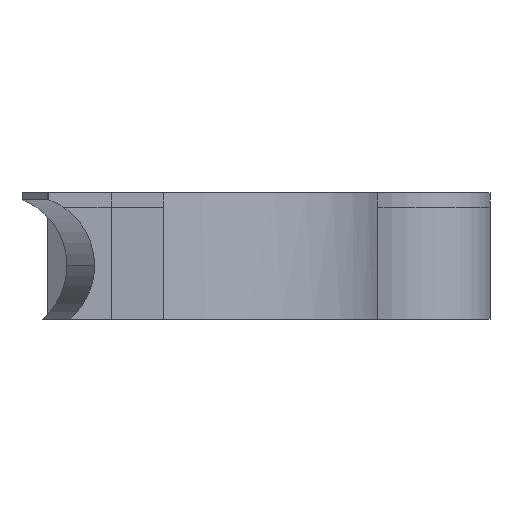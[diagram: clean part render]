
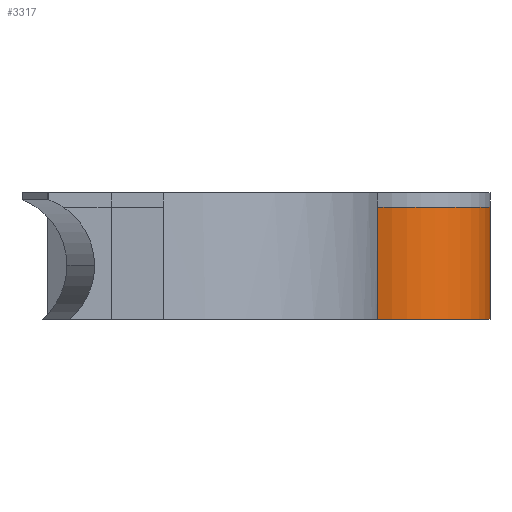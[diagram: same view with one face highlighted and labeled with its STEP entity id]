
A CAD part, left-side view. The second image highlights one B-rep face of the part: STEP entity #3317.
In plain terms, the highlighted cylindrical face has radius 6 mm (diameter 12 mm), a partial arc.
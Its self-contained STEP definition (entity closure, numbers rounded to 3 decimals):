
#795 = VERTEX_POINT('',#796);
#796 = CARTESIAN_POINT('',(42.343,0.,0.)
  );
#847 = PLANE('',#848);
#848 = AXIS2_PLACEMENT_3D('',#849,#850,#851);
#849 = CARTESIAN_POINT('',(0.,0.,0.));
#850 = DIRECTION('',(0.,1.,0.));
#851 = DIRECTION('',(1.,0.,0.));
#1685 = VERTEX_POINT('',#1686);
#1686 = CARTESIAN_POINT('',(42.343,0.,8.));
#1707 = EDGE_CURVE('',#795,#1685,#1708,.T.);
#1708 = SURFACE_CURVE('',#1709,(#1713,#1719),.PCURVE_S1.);
#1709 = LINE('',#1710,#1711);
#1710 = CARTESIAN_POINT('',(42.343,0.,8.));
#1711 = VECTOR('',#1712,1.);
#1712 = DIRECTION('',(0.,0.,1.));
#1713 = PCURVE('',#847,#1714);
#1714 = DEFINITIONAL_REPRESENTATION('',(#1715),#1718);
#1715 = B_SPLINE_CURVE_WITH_KNOTS('',1,(#1716,#1717),.UNSPECIFIED.,.F.,
  .F.,(2,2),(-8.,0.),.PIECEWISE_BEZIER_KNOTS.);
#1716 = CARTESIAN_POINT('',(42.343,0.));
#1717 = CARTESIAN_POINT('',(42.343,-8.));
#1718 = ( GEOMETRIC_REPRESENTATION_CONTEXT(2) 
PARAMETRIC_REPRESENTATION_CONTEXT() REPRESENTATION_CONTEXT('2D SPACE',''
  ) );
#1719 = PCURVE('',#1720,#1725);
#1720 = CYLINDRICAL_SURFACE('',#1721,6.);
#1721 = AXIS2_PLACEMENT_3D('',#1722,#1723,#1724);
#1722 = CARTESIAN_POINT('',(48.,-2.,8.));
#1723 = DIRECTION('',(0.,0.,1.));
#1724 = DIRECTION('',(1.,0.,0.));
#1725 = DEFINITIONAL_REPRESENTATION('',(#1726),#1729);
#1726 = B_SPLINE_CURVE_WITH_KNOTS('',1,(#1727,#1728),.UNSPECIFIED.,.F.,
  .F.,(2,2),(-8.,0.),.PIECEWISE_BEZIER_KNOTS.);
#1727 = CARTESIAN_POINT('',(2.802,-8.));
#1728 = CARTESIAN_POINT('',(2.802,0.));
#1729 = ( GEOMETRIC_REPRESENTATION_CONTEXT(2) 
PARAMETRIC_REPRESENTATION_CONTEXT() REPRESENTATION_CONTEXT('2D SPACE',''
  ) );
#1843 = PLANE('',#1844);
#1844 = AXIS2_PLACEMENT_3D('',#1845,#1846,#1847);
#1845 = CARTESIAN_POINT('',(54.,-2.,0.));
#1846 = DIRECTION('',(0.,0.,-1.));
#1847 = DIRECTION('',(-1.,0.,0.));
#2028 = CYLINDRICAL_SURFACE('',#2029,6.);
#2029 = AXIS2_PLACEMENT_3D('',#2030,#2031,#2032);
#2030 = CARTESIAN_POINT('',(48.,-2.,8.));
#2031 = DIRECTION('',(0.,0.,1.));
#2032 = DIRECTION('',(1.,0.,0.));
#2433 = CYLINDRICAL_SURFACE('',#2434,6.);
#2434 = AXIS2_PLACEMENT_3D('',#2435,#2436,#2437);
#2435 = CARTESIAN_POINT('',(48.,-2.,8.));
#2436 = DIRECTION('',(0.,0.,-1.));
#2437 = DIRECTION('',(1.,0.,0.));
#3317 = ADVANCED_FACE('',(#3318),#1720,.T.);
#3318 = FACE_BOUND('',#3319,.T.);
#3319 = EDGE_LOOP('',(#3320,#3345,#3367,#3368));
#3320 = ORIENTED_EDGE('',*,*,#3321,.F.);
#3321 = EDGE_CURVE('',#3322,#3324,#3326,.T.);
#3322 = VERTEX_POINT('',#3323);
#3323 = CARTESIAN_POINT('',(54.,-2.,8.));
#3324 = VERTEX_POINT('',#3325);
#3325 = CARTESIAN_POINT('',(54.,-2.,0.));
#3326 = SURFACE_CURVE('',#3327,(#3331,#3338),.PCURVE_S1.);
#3327 = LINE('',#3328,#3329);
#3328 = CARTESIAN_POINT('',(54.,-2.,8.));
#3329 = VECTOR('',#3330,1.);
#3330 = DIRECTION('',(0.,0.,-1.));
#3331 = PCURVE('',#1720,#3332);
#3332 = DEFINITIONAL_REPRESENTATION('',(#3333),#3337);
#3333 = LINE('',#3334,#3335);
#3334 = CARTESIAN_POINT('',(6.283,0.));
#3335 = VECTOR('',#3336,1.);
#3336 = DIRECTION('',(0.,-1.));
#3337 = ( GEOMETRIC_REPRESENTATION_CONTEXT(2) 
PARAMETRIC_REPRESENTATION_CONTEXT() REPRESENTATION_CONTEXT('2D SPACE',''
  ) );
#3338 = PCURVE('',#2028,#3339);
#3339 = DEFINITIONAL_REPRESENTATION('',(#3340),#3344);
#3340 = LINE('',#3341,#3342);
#3341 = CARTESIAN_POINT('',(0.,0.));
#3342 = VECTOR('',#3343,1.);
#3343 = DIRECTION('',(0.,-1.));
#3344 = ( GEOMETRIC_REPRESENTATION_CONTEXT(2) 
PARAMETRIC_REPRESENTATION_CONTEXT() REPRESENTATION_CONTEXT('2D SPACE',''
  ) );
#3345 = ORIENTED_EDGE('',*,*,#3346,.F.);
#3346 = EDGE_CURVE('',#1685,#3322,#3347,.T.);
#3347 = SURFACE_CURVE('',#3348,(#3353,#3360),.PCURVE_S1.);
#3348 = CIRCLE('',#3349,6.);
#3349 = AXIS2_PLACEMENT_3D('',#3350,#3351,#3352);
#3350 = CARTESIAN_POINT('',(48.,-2.,8.));
#3351 = DIRECTION('',(0.,0.,1.));
#3352 = DIRECTION('',(1.,0.,0.));
#3353 = PCURVE('',#1720,#3354);
#3354 = DEFINITIONAL_REPRESENTATION('',(#3355),#3359);
#3355 = LINE('',#3356,#3357);
#3356 = CARTESIAN_POINT('',(0.,0.));
#3357 = VECTOR('',#3358,1.);
#3358 = DIRECTION('',(1.,0.));
#3359 = ( GEOMETRIC_REPRESENTATION_CONTEXT(2) 
PARAMETRIC_REPRESENTATION_CONTEXT() REPRESENTATION_CONTEXT('2D SPACE',''
  ) );
#3360 = PCURVE('',#2433,#3361);
#3361 = DEFINITIONAL_REPRESENTATION('',(#3362),#3366);
#3362 = LINE('',#3363,#3364);
#3363 = CARTESIAN_POINT('',(0.,0.));
#3364 = VECTOR('',#3365,1.);
#3365 = DIRECTION('',(-1.,0.));
#3366 = ( GEOMETRIC_REPRESENTATION_CONTEXT(2) 
PARAMETRIC_REPRESENTATION_CONTEXT() REPRESENTATION_CONTEXT('2D SPACE',''
  ) );
#3367 = ORIENTED_EDGE('',*,*,#1707,.F.);
#3368 = ORIENTED_EDGE('',*,*,#3369,.T.);
#3369 = EDGE_CURVE('',#795,#3324,#3370,.T.);
#3370 = SURFACE_CURVE('',#3371,(#3376,#3383),.PCURVE_S1.);
#3371 = CIRCLE('',#3372,6.);
#3372 = AXIS2_PLACEMENT_3D('',#3373,#3374,#3375);
#3373 = CARTESIAN_POINT('',(48.,-2.,0.));
#3374 = DIRECTION('',(0.,0.,1.));
#3375 = DIRECTION('',(1.,0.,0.));
#3376 = PCURVE('',#1720,#3377);
#3377 = DEFINITIONAL_REPRESENTATION('',(#3378),#3382);
#3378 = LINE('',#3379,#3380);
#3379 = CARTESIAN_POINT('',(0.,-8.));
#3380 = VECTOR('',#3381,1.);
#3381 = DIRECTION('',(1.,0.));
#3382 = ( GEOMETRIC_REPRESENTATION_CONTEXT(2) 
PARAMETRIC_REPRESENTATION_CONTEXT() REPRESENTATION_CONTEXT('2D SPACE',''
  ) );
#3383 = PCURVE('',#1843,#3384);
#3384 = DEFINITIONAL_REPRESENTATION('',(#3385),#3393);
#3385 = ( BOUNDED_CURVE() B_SPLINE_CURVE(2,(#3386,#3387,#3388,#3389,
#3390,#3391,#3392),.UNSPECIFIED.,.F.,.F.) B_SPLINE_CURVE_WITH_KNOTS((1,2
    ,2,2,2,1),(-2.094,0.,2.094,4.189,
6.283,8.378),.UNSPECIFIED.) CURVE() 
GEOMETRIC_REPRESENTATION_ITEM() RATIONAL_B_SPLINE_CURVE((1.,0.5,1.,0.5,
1.,0.5,1.)) REPRESENTATION_ITEM('') );
#3386 = CARTESIAN_POINT('',(0.,0.));
#3387 = CARTESIAN_POINT('',(0.,10.392));
#3388 = CARTESIAN_POINT('',(9.,5.196));
#3389 = CARTESIAN_POINT('',(18.,0.));
#3390 = CARTESIAN_POINT('',(9.,-5.196));
#3391 = CARTESIAN_POINT('',(0.,-10.392));
#3392 = CARTESIAN_POINT('',(0.,0.));
#3393 = ( GEOMETRIC_REPRESENTATION_CONTEXT(2) 
PARAMETRIC_REPRESENTATION_CONTEXT() REPRESENTATION_CONTEXT('2D SPACE',''
  ) );
